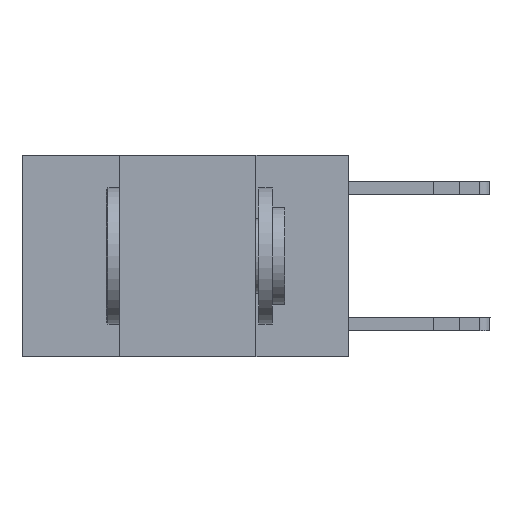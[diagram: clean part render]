
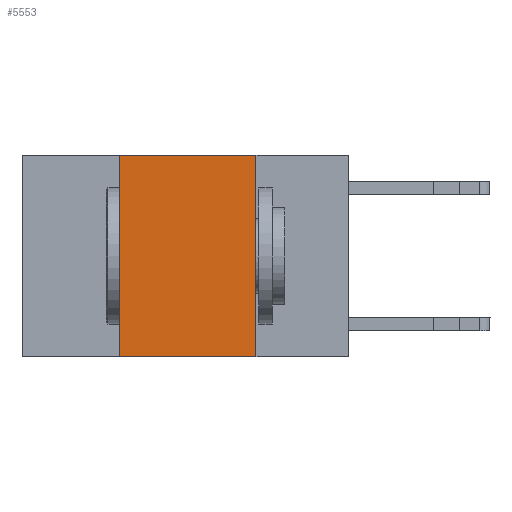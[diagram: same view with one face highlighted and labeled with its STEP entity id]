
A CAD part, left-side view. The second image highlights one B-rep face of the part: STEP entity #5553.
In plain terms, the highlighted planar face has unit normal (-1, 0, 0).
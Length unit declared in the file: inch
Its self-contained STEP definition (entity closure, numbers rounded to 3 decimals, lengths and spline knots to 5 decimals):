
#946 = VECTOR ( 'NONE', #12885, 39.37008 ) ;
#983 = CARTESIAN_POINT ( 'NONE',  ( 0., 0.17, 0. ) ) ;
#1745 = CARTESIAN_POINT ( 'NONE',  ( 0., 0.6, -0.37 ) ) ;
#2361 = PLANE ( 'NONE',  #11580 ) ;
#2758 = VERTEX_POINT ( 'NONE', #8080 ) ;
#3644 = VERTEX_POINT ( 'NONE', #5757 ) ;
#4537 = VERTEX_POINT ( 'NONE', #14945 ) ;
#4561 = DIRECTION ( 'NONE',  ( 0., 0., -1. ) ) ;
#5148 = LINE ( 'NONE', #6856, #11516 ) ;
#5502 = ORIENTED_EDGE ( 'NONE', *, *, #15211, .F. ) ;
#5553 = ADVANCED_FACE ( 'NONE', ( #14410 ), #2361, .F. ) ;
#5757 = CARTESIAN_POINT ( 'NONE',  ( 0., 0.17, -0.37 ) ) ;
#6184 = DIRECTION ( 'NONE',  ( 1., 0., 0. ) ) ;
#6856 = CARTESIAN_POINT ( 'NONE',  ( 0., 0.42, 0. ) ) ;
#8080 = CARTESIAN_POINT ( 'NONE',  ( 0., 0.42, 0. ) ) ;
#8205 = CARTESIAN_POINT ( 'NONE',  ( 0., 0.6, 0. ) ) ;
#8964 = VECTOR ( 'NONE', #9172, 39.37008 ) ;
#9172 = DIRECTION ( 'NONE',  ( 0., -1., 0. ) ) ;
#9198 = VERTEX_POINT ( 'NONE', #983 ) ;
#9758 = CARTESIAN_POINT ( 'NONE',  ( 0., 0.6, 0. ) ) ;
#9822 = ORIENTED_EDGE ( 'NONE', *, *, #14335, .T. ) ;
#9874 = VECTOR ( 'NONE', #4561, 39.37008 ) ;
#9896 = EDGE_LOOP ( 'NONE', ( #12470, #5502, #15528, #9822 ) ) ;
#10417 = LINE ( 'NONE', #8205, #946 ) ;
#11516 = VECTOR ( 'NONE', #11567, 39.37008 ) ;
#11567 = DIRECTION ( 'NONE',  ( 0., 0., 1. ) ) ;
#11580 = AXIS2_PLACEMENT_3D ( 'NONE', #9758, #6184, #14413 ) ;
#12015 = EDGE_CURVE ( 'NONE', #9198, #3644, #12587, .T. ) ;
#12450 = LINE ( 'NONE', #1745, #8964 ) ;
#12470 = ORIENTED_EDGE ( 'NONE', *, *, #12015, .F. ) ;
#12587 = LINE ( 'NONE', #12908, #9874 ) ;
#12885 = DIRECTION ( 'NONE',  ( 0., -1., 0. ) ) ;
#12908 = CARTESIAN_POINT ( 'NONE',  ( 0., 0.17, 0. ) ) ;
#14335 = EDGE_CURVE ( 'NONE', #4537, #3644, #12450, .T. ) ;
#14410 = FACE_OUTER_BOUND ( 'NONE', #9896, .T. ) ;
#14413 = DIRECTION ( 'NONE',  ( 0., 0., -1. ) ) ;
#14945 = CARTESIAN_POINT ( 'NONE',  ( 0., 0.42, -0.37 ) ) ;
#15103 = EDGE_CURVE ( 'NONE', #4537, #2758, #5148, .T. ) ;
#15211 = EDGE_CURVE ( 'NONE', #2758, #9198, #10417, .T. ) ;
#15528 = ORIENTED_EDGE ( 'NONE', *, *, #15103, .F. ) ;
